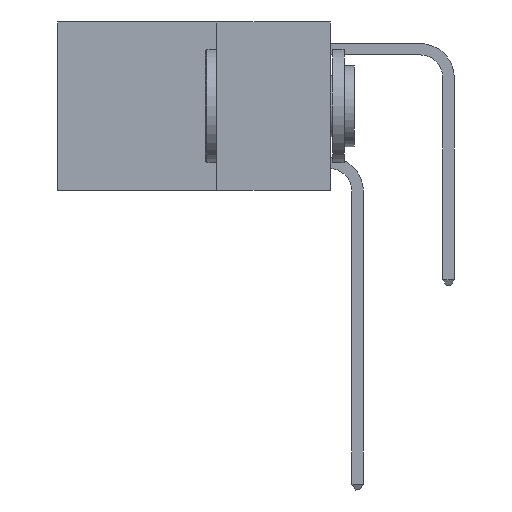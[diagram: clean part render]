
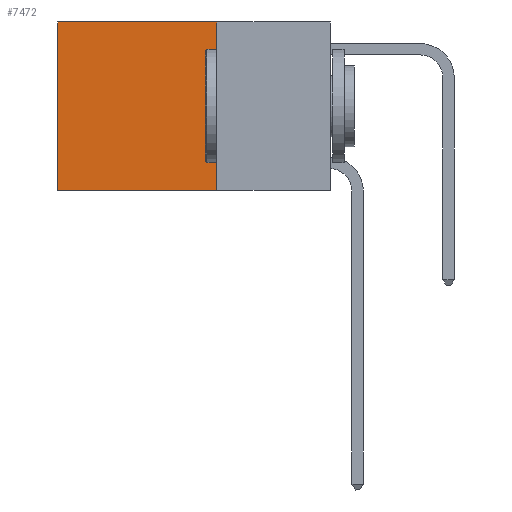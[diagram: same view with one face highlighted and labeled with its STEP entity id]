
A CAD part, left-side view. The second image highlights one B-rep face of the part: STEP entity #7472.
In plain terms, the highlighted planar face has unit normal (-1, 0, 0).
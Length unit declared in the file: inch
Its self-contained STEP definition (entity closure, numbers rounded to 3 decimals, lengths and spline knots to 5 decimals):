
#579 = DIRECTION ( 'NONE',  ( 0., 0., -1. ) ) ;
#994 = EDGE_CURVE ( 'NONE', #2751, #4769, #11581, .T. ) ;
#1202 = CARTESIAN_POINT ( 'NONE',  ( 0.2625, 0.25, 0. ) ) ;
#1340 = DIRECTION ( 'NONE',  ( 0., 1., 0. ) ) ;
#1382 = EDGE_LOOP ( 'NONE', ( #10196, #7945, #3988, #5747 ) ) ;
#2147 = CARTESIAN_POINT ( 'NONE',  ( 0.2625, 0.6, 0. ) ) ;
#2245 = EDGE_CURVE ( 'NONE', #7306, #2751, #8680, .T. ) ;
#2325 = EDGE_CURVE ( 'NONE', #5891, #4769, #12320, .T. ) ;
#2625 = DIRECTION ( 'NONE',  ( 1., 0., 0. ) ) ;
#2751 = VERTEX_POINT ( 'NONE', #6672 ) ;
#2855 = CARTESIAN_POINT ( 'NONE',  ( 0.2625, 0.25, 0. ) ) ;
#3170 = AXIS2_PLACEMENT_3D ( 'NONE', #4898, #2625, #12883 ) ;
#3722 = CARTESIAN_POINT ( 'NONE',  ( 0.2625, 0.25, 0. ) ) ;
#3988 = ORIENTED_EDGE ( 'NONE', *, *, #2245, .F. ) ;
#4769 = VERTEX_POINT ( 'NONE', #11989 ) ;
#4840 = LINE ( 'NONE', #3722, #6985 ) ;
#4898 = CARTESIAN_POINT ( 'NONE',  ( 0.2625, 0.25, 0. ) ) ;
#5649 = DIRECTION ( 'NONE',  ( 0., 1., 0. ) ) ;
#5747 = ORIENTED_EDGE ( 'NONE', *, *, #6980, .T. ) ;
#5891 = VERTEX_POINT ( 'NONE', #13356 ) ;
#6672 = CARTESIAN_POINT ( 'NONE',  ( 0.2625, 0.25, -0.37 ) ) ;
#6690 = VECTOR ( 'NONE', #579, 39.37008 ) ;
#6749 = DIRECTION ( 'NONE',  ( 0., 0., -1. ) ) ;
#6980 = EDGE_CURVE ( 'NONE', #7306, #5891, #4840, .T. ) ;
#6985 = VECTOR ( 'NONE', #5649, 39.37008 ) ;
#7306 = VERTEX_POINT ( 'NONE', #1202 ) ;
#7472 = ADVANCED_FACE ( 'NONE', ( #13023 ), #10562, .F. ) ;
#7945 = ORIENTED_EDGE ( 'NONE', *, *, #994, .F. ) ;
#8237 = CARTESIAN_POINT ( 'NONE',  ( 0.2625, 0.25, -0.37 ) ) ;
#8680 = LINE ( 'NONE', #2855, #6690 ) ;
#10196 = ORIENTED_EDGE ( 'NONE', *, *, #2325, .T. ) ;
#10562 = PLANE ( 'NONE',  #3170 ) ;
#11581 = LINE ( 'NONE', #8237, #12121 ) ;
#11989 = CARTESIAN_POINT ( 'NONE',  ( 0.2625, 0.6, -0.37 ) ) ;
#12121 = VECTOR ( 'NONE', #1340, 39.37008 ) ;
#12320 = LINE ( 'NONE', #2147, #13124 ) ;
#12883 = DIRECTION ( 'NONE',  ( 0., 0., -1. ) ) ;
#13023 = FACE_OUTER_BOUND ( 'NONE', #1382, .T. ) ;
#13124 = VECTOR ( 'NONE', #6749, 39.37008 ) ;
#13356 = CARTESIAN_POINT ( 'NONE',  ( 0.2625, 0.6, 0. ) ) ;
